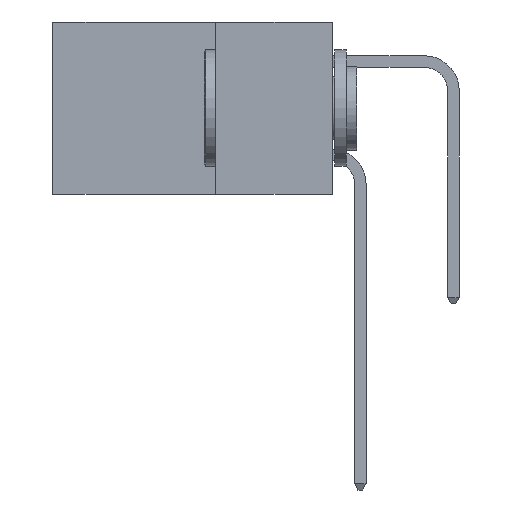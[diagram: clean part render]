
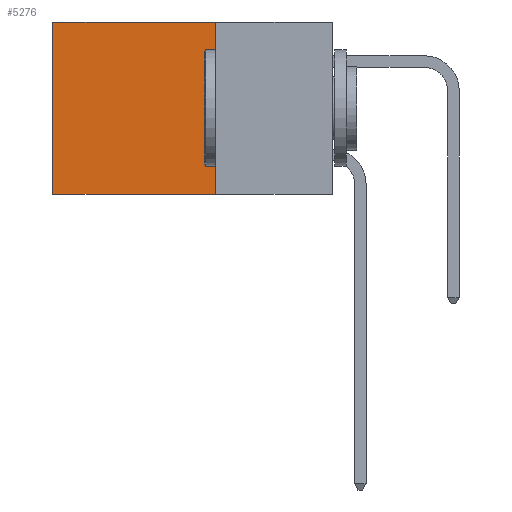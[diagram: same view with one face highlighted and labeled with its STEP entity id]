
A CAD part, left-side view. The second image highlights one B-rep face of the part: STEP entity #5276.
In plain terms, the highlighted planar face has unit normal (-1, 0, 0).
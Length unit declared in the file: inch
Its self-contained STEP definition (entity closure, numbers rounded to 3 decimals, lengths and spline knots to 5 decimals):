
#84 = ORIENTED_EDGE ( 'NONE', *, *, #709, .F. ) ;
#415 = EDGE_CURVE ( 'NONE', #5652, #2817, #17569, .T. ) ;
#709 = EDGE_CURVE ( 'NONE', #2817, #16441, #13304, .T. ) ;
#878 = DIRECTION ( 'NONE',  ( 0., 0., -1. ) ) ;
#1355 = VECTOR ( 'NONE', #12208, 39.37008 ) ;
#2361 = CARTESIAN_POINT ( 'NONE',  ( 0.2615, 0.25, -0.37 ) ) ;
#2817 = VERTEX_POINT ( 'NONE', #2361 ) ;
#3606 = ORIENTED_EDGE ( 'NONE', *, *, #12141, .T. ) ;
#3618 = VECTOR ( 'NONE', #5234, 39.37008 ) ;
#5151 = CARTESIAN_POINT ( 'NONE',  ( 0.2615, 0.6, -0.37 ) ) ;
#5234 = DIRECTION ( 'NONE',  ( 0., 0., -1. ) ) ;
#5276 = ADVANCED_FACE ( 'NONE', ( #11850 ), #7214, .F. ) ;
#5652 = VERTEX_POINT ( 'NONE', #7823 ) ;
#5953 = VERTEX_POINT ( 'NONE', #9329 ) ;
#6111 = VECTOR ( 'NONE', #16244, 39.37008 ) ;
#6754 = VECTOR ( 'NONE', #878, 39.37008 ) ;
#7023 = EDGE_LOOP ( 'NONE', ( #3606, #84, #13947, #8082 ) ) ;
#7214 = PLANE ( 'NONE',  #8644 ) ;
#7591 = DIRECTION ( 'NONE',  ( 1., 0., 0. ) ) ;
#7596 = DIRECTION ( 'NONE',  ( 0., 0., -1. ) ) ;
#7626 = CARTESIAN_POINT ( 'NONE',  ( 0.2615, 0.25, -0.37 ) ) ;
#7823 = CARTESIAN_POINT ( 'NONE',  ( 0.2615, 0.25, 0. ) ) ;
#8082 = ORIENTED_EDGE ( 'NONE', *, *, #15231, .T. ) ;
#8644 = AXIS2_PLACEMENT_3D ( 'NONE', #7626, #7591, #7596 ) ;
#9118 = LINE ( 'NONE', #10886, #1355 ) ;
#9329 = CARTESIAN_POINT ( 'NONE',  ( 0.2615, 0.6, 0. ) ) ;
#10483 = LINE ( 'NONE', #5151, #3618 ) ;
#10886 = CARTESIAN_POINT ( 'NONE',  ( 0.2615, 0.25, 0. ) ) ;
#11850 = FACE_OUTER_BOUND ( 'NONE', #7023, .T. ) ;
#12141 = EDGE_CURVE ( 'NONE', #5953, #16441, #10483, .T. ) ;
#12208 = DIRECTION ( 'NONE',  ( 0., 1., 0. ) ) ;
#12610 = CARTESIAN_POINT ( 'NONE',  ( 0.2615, 0.25, -0.37 ) ) ;
#13218 = CARTESIAN_POINT ( 'NONE',  ( 0.2615, 0.6, -0.37 ) ) ;
#13304 = LINE ( 'NONE', #12610, #6111 ) ;
#13947 = ORIENTED_EDGE ( 'NONE', *, *, #415, .F. ) ;
#14255 = CARTESIAN_POINT ( 'NONE',  ( 0.2615, 0.25, -0.37 ) ) ;
#15231 = EDGE_CURVE ( 'NONE', #5652, #5953, #9118, .T. ) ;
#16244 = DIRECTION ( 'NONE',  ( 0., 1., 0. ) ) ;
#16441 = VERTEX_POINT ( 'NONE', #13218 ) ;
#17569 = LINE ( 'NONE', #14255, #6754 ) ;
